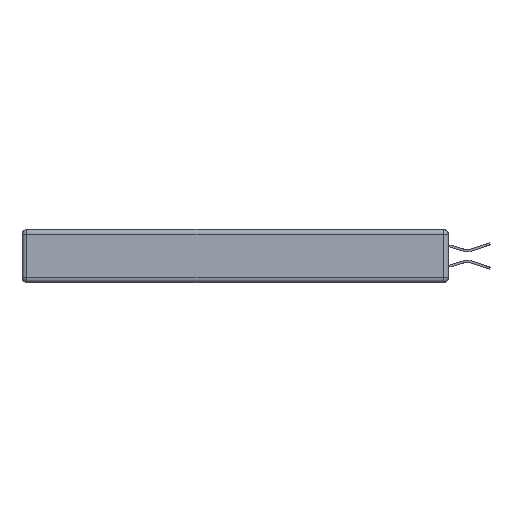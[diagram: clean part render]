
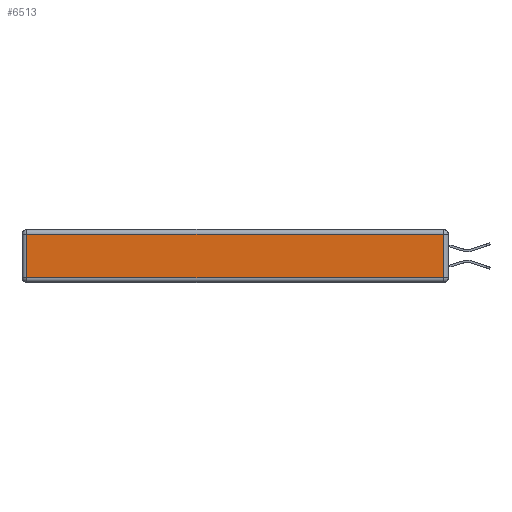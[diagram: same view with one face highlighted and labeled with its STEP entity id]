
A CAD part, left-side view. The second image highlights one B-rep face of the part: STEP entity #6513.
In plain terms, the highlighted planar face has unit normal (-1, 0, 0).
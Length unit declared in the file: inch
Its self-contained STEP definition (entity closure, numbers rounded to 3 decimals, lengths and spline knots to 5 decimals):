
#551 = ORIENTED_EDGE ( 'NONE', *, *, #7352, .T. ) ;
#730 = LINE ( 'NONE', #17575, #13418 ) ;
#967 = DIRECTION ( 'NONE',  ( 0., -1., 0. ) ) ;
#1084 = VERTEX_POINT ( 'NONE', #9196 ) ;
#2118 = ORIENTED_EDGE ( 'NONE', *, *, #24830, .T. ) ;
#2315 = DIRECTION ( 'NONE',  ( -1., 0., 0. ) ) ;
#2550 = CARTESIAN_POINT ( 'NONE',  ( 0., 0., -0.313 ) ) ;
#3825 = DIRECTION ( 'NONE',  ( 0., 1., 0. ) ) ;
#4464 = CARTESIAN_POINT ( 'NONE',  ( 0., 0.03, -0.313 ) ) ;
#4796 = DIRECTION ( 'NONE',  ( 0., 0., -1. ) ) ;
#6136 = EDGE_LOOP ( 'NONE', ( #551, #2118, #8618, #20954 ) ) ;
#6513 = ADVANCED_FACE ( 'NONE', ( #23199 ), #23140, .T. ) ;
#7352 = EDGE_CURVE ( 'NONE', #1084, #23923, #11005, .T. ) ;
#7379 = CARTESIAN_POINT ( 'NONE',  ( 0., 2.72, -0.03 ) ) ;
#8618 = ORIENTED_EDGE ( 'NONE', *, *, #9351, .T. ) ;
#9196 = CARTESIAN_POINT ( 'NONE',  ( 0., 2.72, -0.313 ) ) ;
#9351 = EDGE_CURVE ( 'NONE', #21818, #21329, #21641, .T. ) ;
#9911 = VECTOR ( 'NONE', #3825, 39.37008 ) ;
#11005 = LINE ( 'NONE', #2550, #11324 ) ;
#11324 = VECTOR ( 'NONE', #967, 39.37008 ) ;
#13418 = VECTOR ( 'NONE', #4796, 39.37008 ) ;
#14051 = AXIS2_PLACEMENT_3D ( 'NONE', #25310, #2315, #23606 ) ;
#15071 = CARTESIAN_POINT ( 'NONE',  ( 0., 0.03, -0.03 ) ) ;
#16149 = EDGE_CURVE ( 'NONE', #21329, #1084, #730, .T. ) ;
#16552 = CARTESIAN_POINT ( 'NONE',  ( 0., 2.75, -0.03 ) ) ;
#16734 = VECTOR ( 'NONE', #25406, 39.37008 ) ;
#17575 = CARTESIAN_POINT ( 'NONE',  ( 0., 2.72, -0.343 ) ) ;
#19498 = LINE ( 'NONE', #27663, #16734 ) ;
#20954 = ORIENTED_EDGE ( 'NONE', *, *, #16149, .T. ) ;
#21329 = VERTEX_POINT ( 'NONE', #7379 ) ;
#21641 = LINE ( 'NONE', #16552, #9911 ) ;
#21818 = VERTEX_POINT ( 'NONE', #15071 ) ;
#23140 = PLANE ( 'NONE',  #14051 ) ;
#23199 = FACE_OUTER_BOUND ( 'NONE', #6136, .T. ) ;
#23606 = DIRECTION ( 'NONE',  ( 0., 0., 1. ) ) ;
#23923 = VERTEX_POINT ( 'NONE', #4464 ) ;
#24830 = EDGE_CURVE ( 'NONE', #23923, #21818, #19498, .T. ) ;
#25310 = CARTESIAN_POINT ( 'NONE',  ( 0., 0., -0.343 ) ) ;
#25406 = DIRECTION ( 'NONE',  ( 0., 0., 1. ) ) ;
#27663 = CARTESIAN_POINT ( 'NONE',  ( 0., 0.03, -0.343 ) ) ;
